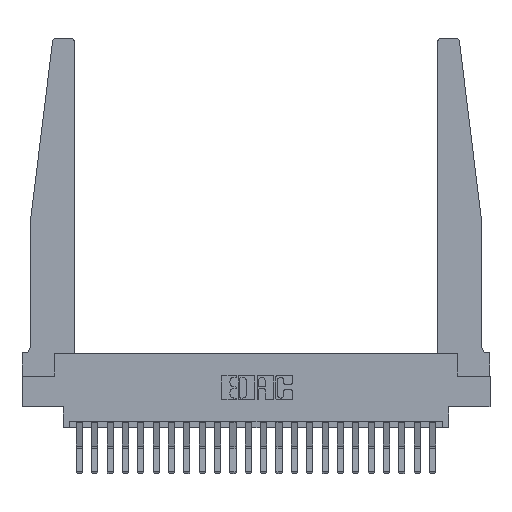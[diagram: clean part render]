
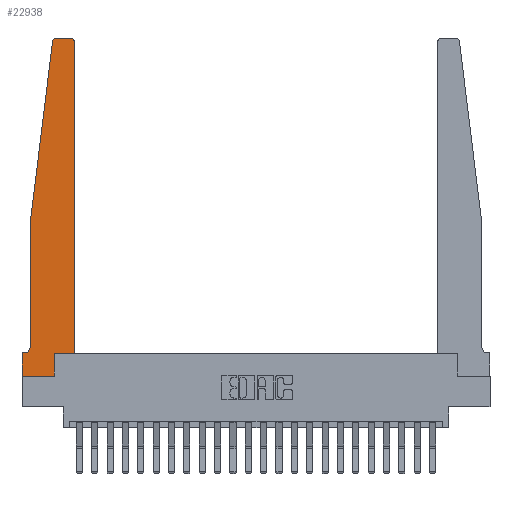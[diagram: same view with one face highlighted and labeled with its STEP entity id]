
A CAD part, top view. The second image highlights one B-rep face of the part: STEP entity #22938.
In plain terms, the highlighted planar face has unit normal (0, 0, 1).
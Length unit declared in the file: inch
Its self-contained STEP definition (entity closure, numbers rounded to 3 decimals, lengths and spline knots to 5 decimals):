
#45 = DIRECTION ( 'NONE',  ( 1., 0., 0. ) ) ;
#654 = ORIENTED_EDGE ( 'NONE', *, *, #5716, .T. ) ;
#817 = VERTEX_POINT ( 'NONE', #4396 ) ;
#1507 = CARTESIAN_POINT ( 'NONE',  ( 0.065, 0.1875, 0.37 ) ) ;
#1746 = VERTEX_POINT ( 'NONE', #10828 ) ;
#1767 = FACE_OUTER_BOUND ( 'NONE', #13498, .T. ) ;
#2438 = ORIENTED_EDGE ( 'NONE', *, *, #20406, .T. ) ;
#3002 = EDGE_CURVE ( 'NONE', #19233, #1746, #22459, .T. ) ;
#3469 = DIRECTION ( 'NONE',  ( 0., 1., 0. ) ) ;
#3743 = CARTESIAN_POINT ( 'NONE',  ( 0.27653, 2.72, 0.37 ) ) ;
#4113 = VECTOR ( 'NONE', #15211, 39.37008 ) ;
#4368 = LINE ( 'NONE', #16925, #17511 ) ;
#4396 = CARTESIAN_POINT ( 'NONE',  ( 0., 0.1875, 0.37 ) ) ;
#4535 = DIRECTION ( 'NONE',  ( 0., 1., 0. ) ) ;
#5552 = DIRECTION ( 'NONE',  ( 1., 0., 0. ) ) ;
#5650 = CARTESIAN_POINT ( 'NONE',  ( 0.015, 0.2375, 0.37 ) ) ;
#5716 = EDGE_CURVE ( 'NONE', #1746, #16355, #15434, .T. ) ;
#5909 = AXIS2_PLACEMENT_3D ( 'NONE', #18292, #7610, #20080 ) ;
#6061 = VECTOR ( 'NONE', #4535, 39.37008 ) ;
#6272 = ORIENTED_EDGE ( 'NONE', *, *, #20113, .T. ) ;
#6389 = ORIENTED_EDGE ( 'NONE', *, *, #9578, .T. ) ;
#6400 = CARTESIAN_POINT ( 'NONE',  ( 0.425, 0.18, 0.37 ) ) ;
#6577 = DIRECTION ( 'NONE',  ( 0., -1., 0. ) ) ;
#6770 = CARTESIAN_POINT ( 'NONE',  ( 0.425, 2.72, 0.37 ) ) ;
#7087 = VECTOR ( 'NONE', #6577, 39.37008 ) ;
#7451 = VERTEX_POINT ( 'NONE', #6770 ) ;
#7464 = DIRECTION ( 'NONE',  ( -1., 0., 0. ) ) ;
#7610 = DIRECTION ( 'NONE',  ( 0., 0., 1. ) ) ;
#7755 = VECTOR ( 'NONE', #10404, 39.37008 ) ;
#8198 = LINE ( 'NONE', #15479, #7087 ) ;
#8517 = DIRECTION ( 'NONE',  ( 0., 0., 1. ) ) ;
#8972 = EDGE_CURVE ( 'NONE', #817, #21987, #18370, .T. ) ;
#9149 = VECTOR ( 'NONE', #3469, 39.37008 ) ;
#9235 = EDGE_CURVE ( 'NONE', #16664, #19233, #17534, .T. ) ;
#9530 = AXIS2_PLACEMENT_3D ( 'NONE', #19194, #8517, #20987 ) ;
#9578 = EDGE_CURVE ( 'NONE', #17770, #7451, #11358, .T. ) ;
#10096 = ORIENTED_EDGE ( 'NONE', *, *, #9235, .T. ) ;
#10404 = DIRECTION ( 'NONE',  ( -1., 0., 0. ) ) ;
#10426 = CARTESIAN_POINT ( 'NONE',  ( 0.065, 0.2375, 0.37 ) ) ;
#10482 = ORIENTED_EDGE ( 'NONE', *, *, #8972, .T. ) ;
#10722 = CARTESIAN_POINT ( 'NONE',  ( 0., 0., 0.37 ) ) ;
#10804 = AXIS2_PLACEMENT_3D ( 'NONE', #3743, #16271, #5552 ) ;
#10828 = CARTESIAN_POINT ( 'NONE',  ( 0.24675, 2.72367, 0.37 ) ) ;
#11230 = CARTESIAN_POINT ( 'NONE',  ( 0.395, 2.75, 0.37 ) ) ;
#11358 = LINE ( 'NONE', #16978, #6061 ) ;
#11519 = CARTESIAN_POINT ( 'NONE',  ( 0.065, 1.25, 0.37 ) ) ;
#11585 = CARTESIAN_POINT ( 'NONE',  ( 0.2605, 0., 0.37 ) ) ;
#11596 = DIRECTION ( 'NONE',  ( -0.122, -0.992, 0. ) ) ;
#11946 = LINE ( 'NONE', #1507, #7755 ) ;
#12214 = CARTESIAN_POINT ( 'NONE',  ( 0.2605, 0.18, 0.37 ) ) ;
#13093 = CIRCLE ( 'NONE', #22726, 0.05 ) ;
#13412 = CARTESIAN_POINT ( 'NONE',  ( 0., 0., 0.37 ) ) ;
#13498 = EDGE_LOOP ( 'NONE', ( #10096, #21068, #654, #17200, #16416, #2438, #10482, #16798, #19630, #15050, #6389, #6272 ) ) ;
#13543 = EDGE_CURVE ( 'NONE', #21784, #17543, #13093, .T. ) ;
#14481 = LINE ( 'NONE', #19575, #9149 ) ;
#15050 = ORIENTED_EDGE ( 'NONE', *, *, #15422, .T. ) ;
#15211 = DIRECTION ( 'NONE',  ( 0., -1., 0. ) ) ;
#15422 = EDGE_CURVE ( 'NONE', #22475, #17770, #4368, .T. ) ;
#15434 = LINE ( 'NONE', #11519, #19039 ) ;
#15479 = CARTESIAN_POINT ( 'NONE',  ( 0.065, 1.25, 0.37 ) ) ;
#15628 = PLANE ( 'NONE',  #9530 ) ;
#16158 = LINE ( 'NONE', #10722, #20317 ) ;
#16271 = DIRECTION ( 'NONE',  ( 0., 0., 1. ) ) ;
#16355 = VERTEX_POINT ( 'NONE', #22861 ) ;
#16416 = ORIENTED_EDGE ( 'NONE', *, *, #13543, .T. ) ;
#16664 = VERTEX_POINT ( 'NONE', #11230 ) ;
#16798 = ORIENTED_EDGE ( 'NONE', *, *, #19937, .T. ) ;
#16925 = CARTESIAN_POINT ( 'NONE',  ( 0.425, 0.18, 0.37 ) ) ;
#16978 = CARTESIAN_POINT ( 'NONE',  ( 0.425, 0.18, 0.37 ) ) ;
#17200 = ORIENTED_EDGE ( 'NONE', *, *, #22869, .T. ) ;
#17511 = VECTOR ( 'NONE', #18695, 39.37008 ) ;
#17524 = VERTEX_POINT ( 'NONE', #11585 ) ;
#17534 = LINE ( 'NONE', #19466, #22819 ) ;
#17538 = CIRCLE ( 'NONE', #5909, 0.03 ) ;
#17543 = VERTEX_POINT ( 'NONE', #20546 ) ;
#17770 = VERTEX_POINT ( 'NONE', #6400 ) ;
#18147 = DIRECTION ( 'NONE',  ( 0., 0., -1. ) ) ;
#18292 = CARTESIAN_POINT ( 'NONE',  ( 0.395, 2.72, 0.37 ) ) ;
#18370 = LINE ( 'NONE', #13412, #4113 ) ;
#18695 = DIRECTION ( 'NONE',  ( 1., 0., 0. ) ) ;
#19039 = VECTOR ( 'NONE', #11596, 39.37008 ) ;
#19194 = CARTESIAN_POINT ( 'NONE',  ( 0., 0.1875, 0.37 ) ) ;
#19233 = VERTEX_POINT ( 'NONE', #21131 ) ;
#19319 = EDGE_CURVE ( 'NONE', #17524, #22475, #14481, .T. ) ;
#19466 = CARTESIAN_POINT ( 'NONE',  ( 0.25, 2.75, 0.37 ) ) ;
#19575 = CARTESIAN_POINT ( 'NONE',  ( 0.2605, 0.18, 0.37 ) ) ;
#19630 = ORIENTED_EDGE ( 'NONE', *, *, #19319, .T. ) ;
#19849 = CARTESIAN_POINT ( 'NONE',  ( 0., 0., 0.37 ) ) ;
#19937 = EDGE_CURVE ( 'NONE', #21987, #17524, #16158, .T. ) ;
#20080 = DIRECTION ( 'NONE',  ( 1., 0., 0. ) ) ;
#20113 = EDGE_CURVE ( 'NONE', #7451, #16664, #17538, .T. ) ;
#20317 = VECTOR ( 'NONE', #45, 39.37008 ) ;
#20406 = EDGE_CURVE ( 'NONE', #17543, #817, #11946, .T. ) ;
#20546 = CARTESIAN_POINT ( 'NONE',  ( 0.015, 0.1875, 0.37 ) ) ;
#20987 = DIRECTION ( 'NONE',  ( 1., 0., 0. ) ) ;
#21068 = ORIENTED_EDGE ( 'NONE', *, *, #3002, .T. ) ;
#21131 = CARTESIAN_POINT ( 'NONE',  ( 0.27653, 2.75, 0.37 ) ) ;
#21251 = DIRECTION ( 'NONE',  ( -1., 0., 0. ) ) ;
#21784 = VERTEX_POINT ( 'NONE', #10426 ) ;
#21987 = VERTEX_POINT ( 'NONE', #19849 ) ;
#22459 = CIRCLE ( 'NONE', #10804, 0.03 ) ;
#22475 = VERTEX_POINT ( 'NONE', #12214 ) ;
#22726 = AXIS2_PLACEMENT_3D ( 'NONE', #5650, #18147, #7464 ) ;
#22819 = VECTOR ( 'NONE', #21251, 39.37008 ) ;
#22861 = CARTESIAN_POINT ( 'NONE',  ( 0.065, 1.25, 0.37 ) ) ;
#22869 = EDGE_CURVE ( 'NONE', #16355, #21784, #8198, .T. ) ;
#22938 = ADVANCED_FACE ( 'NONE', ( #1767 ), #15628, .T. ) ;
